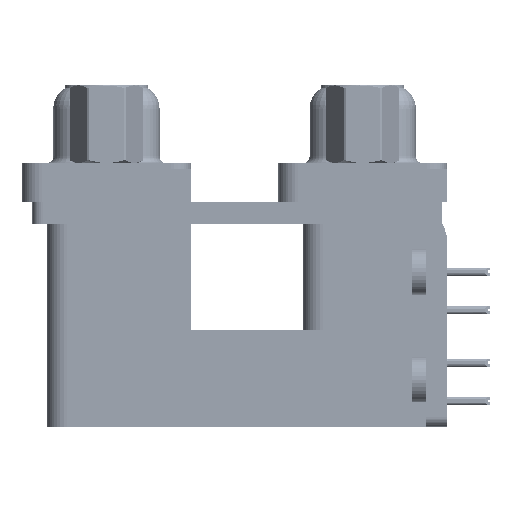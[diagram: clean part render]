
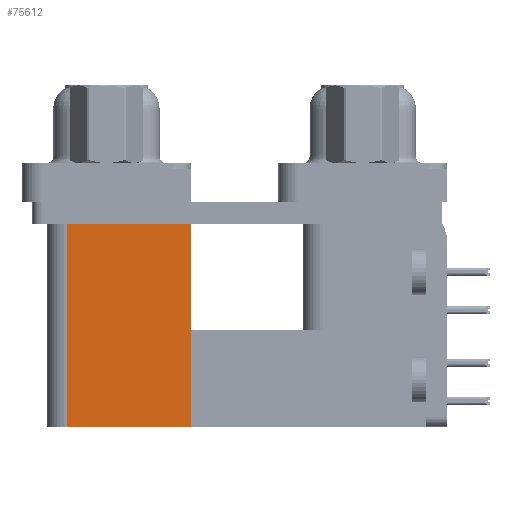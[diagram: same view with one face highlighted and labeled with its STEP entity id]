
A CAD part, left-side view. The second image highlights one B-rep face of the part: STEP entity #75612.
In plain terms, the highlighted planar face has unit normal (-1, 0, 0).
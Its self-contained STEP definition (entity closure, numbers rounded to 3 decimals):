
#156 = CARTESIAN_POINT ( 'NONE',  ( 3.79, 12.775, -2.5 ) ) ;
#347 = DIRECTION ( 'NONE',  ( 0., 0., -1. ) ) ;
#6719 = VERTEX_POINT ( 'NONE', #81520 ) ;
#12312 = FACE_OUTER_BOUND ( 'NONE', #44405, .T. ) ;
#13701 = CARTESIAN_POINT ( 'NONE',  ( 3.79, 12.775, -19.2 ) ) ;
#15025 = ORIENTED_EDGE ( 'NONE', *, *, #41278, .F. ) ;
#16298 = DIRECTION ( 'NONE',  ( 0., 1., 0. ) ) ;
#19758 = PLANE ( 'NONE',  #55199 ) ;
#20033 = VERTEX_POINT ( 'NONE', #42687 ) ;
#22938 = LINE ( 'NONE', #80785, #27170 ) ;
#24708 = ORIENTED_EDGE ( 'NONE', *, *, #74622, .T. ) ;
#27170 = VECTOR ( 'NONE', #16298, 1000. ) ;
#31094 = EDGE_CURVE ( 'NONE', #6719, #20033, #22938, .T. ) ;
#34843 = LINE ( 'NONE', #66718, #79420 ) ;
#37566 = CARTESIAN_POINT ( 'NONE',  ( 3.79, 12.775, -19.2 ) ) ;
#39380 = DIRECTION ( 'NONE',  ( 0., 0., 1. ) ) ;
#39789 = CARTESIAN_POINT ( 'NONE',  ( 3.79, 12.775, -2.5 ) ) ;
#41278 = EDGE_CURVE ( 'NONE', #20033, #51651, #34843, .T. ) ;
#42687 = CARTESIAN_POINT ( 'NONE',  ( 3.79, 21.975, -19.2 ) ) ;
#44405 = EDGE_LOOP ( 'NONE', ( #24708, #15025, #56439, #66170 ) ) ;
#48231 = VERTEX_POINT ( 'NONE', #156 ) ;
#51651 = VERTEX_POINT ( 'NONE', #72490 ) ;
#55199 = AXIS2_PLACEMENT_3D ( 'NONE', #37566, #69413, #347 ) ;
#56439 = ORIENTED_EDGE ( 'NONE', *, *, #31094, .F. ) ;
#57987 = LINE ( 'NONE', #13701, #76364 ) ;
#58414 = DIRECTION ( 'NONE',  ( 0., 1., 0. ) ) ;
#59010 = VECTOR ( 'NONE', #58414, 1000. ) ;
#66170 = ORIENTED_EDGE ( 'NONE', *, *, #73698, .T. ) ;
#66718 = CARTESIAN_POINT ( 'NONE',  ( 3.79, 21.975, -19.2 ) ) ;
#69413 = DIRECTION ( 'NONE',  ( 1., 0., 0. ) ) ;
#72490 = CARTESIAN_POINT ( 'NONE',  ( 3.79, 21.975, -2.5 ) ) ;
#72904 = DIRECTION ( 'NONE',  ( 0., 0., 1. ) ) ;
#73698 = EDGE_CURVE ( 'NONE', #6719, #48231, #57987, .T. ) ;
#74622 = EDGE_CURVE ( 'NONE', #48231, #51651, #79084, .T. ) ;
#75612 = ADVANCED_FACE ( 'NONE', ( #12312 ), #19758, .F. ) ;
#76364 = VECTOR ( 'NONE', #39380, 1000. ) ;
#79084 = LINE ( 'NONE', #39789, #59010 ) ;
#79420 = VECTOR ( 'NONE', #72904, 1000. ) ;
#80785 = CARTESIAN_POINT ( 'NONE',  ( 3.79, 12.775, -19.2 ) ) ;
#81520 = CARTESIAN_POINT ( 'NONE',  ( 3.79, 12.775, -19.2 ) ) ;
